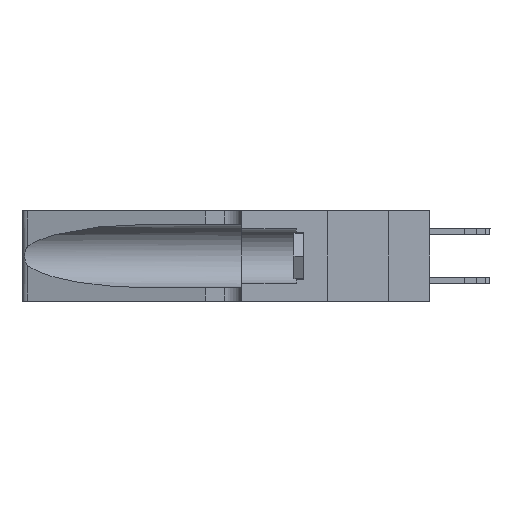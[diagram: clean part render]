
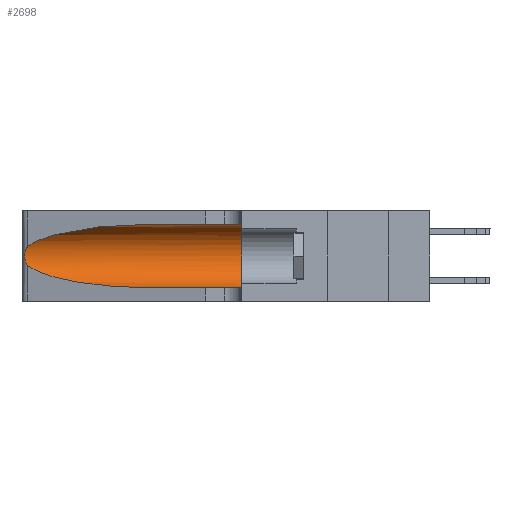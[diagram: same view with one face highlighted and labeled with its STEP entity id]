
A CAD part, left-side view. The second image highlights one B-rep face of the part: STEP entity #2698.
In plain terms, the highlighted cylindrical face has radius 3.308 mm (diameter 6.617 mm), a partial arc.
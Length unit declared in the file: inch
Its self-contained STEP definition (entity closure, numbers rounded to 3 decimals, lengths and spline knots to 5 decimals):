
#829 = CARTESIAN_POINT ( 'NONE',  ( 0.25487, 1.22718, 0.14631 ) ) ;
#1090 = CARTESIAN_POINT ( 'NONE',  ( 0.26075, 1.23896, 0.19203 ) ) ;
#1494 = CARTESIAN_POINT ( 'NONE',  ( 0.18966, 0.96281, 0.31525 ) ) ;
#1847 = VERTEX_POINT ( 'NONE', #18610 ) ;
#1973 = DIRECTION ( 'NONE',  ( 0., 1., 0. ) ) ;
#2018 = ORIENTED_EDGE ( 'NONE', *, *, #15554, .T. ) ;
#2055 = EDGE_CURVE ( 'NONE', #8848, #1847, #17939, .T. ) ;
#2092 = EDGE_CURVE ( 'NONE', #1847, #3056, #12847, .T. ) ;
#2271 =( BOUNDED_CURVE ( )  B_SPLINE_CURVE ( 3, ( #7431, #12796, #12648, #5830 ),
 .UNSPECIFIED., .F., .F. ) 
 B_SPLINE_CURVE_WITH_KNOTS ( ( 4, 4 ),
 ( 3.44316, 4.71239 ),
 .UNSPECIFIED. ) 
 CURVE ( )  GEOMETRIC_REPRESENTATION_ITEM ( )  RATIONAL_B_SPLINE_CURVE ( ( 1., 0.87, 0.87, 1. ) ) 
 REPRESENTATION_ITEM ( '' )  );
#2698 = ADVANCED_FACE ( 'NONE', ( #14183 ), #19706, .F. ) ;
#2825 = ORIENTED_EDGE ( 'NONE', *, *, #3946, .T. ) ;
#3056 = VERTEX_POINT ( 'NONE', #829 ) ;
#3180 = DIRECTION ( 'NONE',  ( 0., -1., 0. ) ) ;
#3276 = CARTESIAN_POINT ( 'NONE',  ( 0.1305, 1.61858, 0.05475 ) ) ;
#3824 = CARTESIAN_POINT ( 'NONE',  ( 0.1305, 0.35, 0.185 ) ) ;
#3946 = EDGE_CURVE ( 'NONE', #22287, #8185, #4849, .T. ) ;
#3987 = VECTOR ( 'NONE', #6839, 39.37008 ) ;
#4849 = LINE ( 'NONE', #3276, #3987 ) ;
#4854 = CARTESIAN_POINT ( 'NONE',  ( 0.25639, 1.23184, 0.21858 ) ) ;
#5127 = AXIS2_PLACEMENT_3D ( 'NONE', #3824, #1973, #7308 ) ;
#5688 = EDGE_LOOP ( 'NONE', ( #17604, #20027, #2018, #2825, #14156, #18607 ) ) ;
#5733 = CARTESIAN_POINT ( 'NONE',  ( 0.25487, 1.22718, 0.22369 ) ) ;
#5830 = CARTESIAN_POINT ( 'NONE',  ( 0.1305, 0.72297, 0.05475 ) ) ;
#6083 = CARTESIAN_POINT ( 'NONE',  ( 0.1305, 0.35, 0.05475 ) ) ;
#6839 = DIRECTION ( 'NONE',  ( 0., -1., 0. ) ) ;
#7308 = DIRECTION ( 'NONE',  ( 0., 0., 1. ) ) ;
#7431 = CARTESIAN_POINT ( 'NONE',  ( 0.25487, 1.22718, 0.14631 ) ) ;
#7936 = LINE ( 'NONE', #16104, #18364 ) ;
#8185 = VERTEX_POINT ( 'NONE', #6083 ) ;
#8848 = VERTEX_POINT ( 'NONE', #9189 ) ;
#9189 = CARTESIAN_POINT ( 'NONE',  ( 0.1305, 0.72297, 0.31525 ) ) ;
#9235 = DIRECTION ( 'NONE',  ( 0., -1., 0. ) ) ;
#9632 = CARTESIAN_POINT ( 'NONE',  ( 0.25555, 1.22994, 0.2215 ) ) ;
#9934 = VERTEX_POINT ( 'NONE', #15305 ) ;
#10336 = CARTESIAN_POINT ( 'NONE',  ( 0.1305, 1.61858, 0.185 ) ) ;
#10504 = CARTESIAN_POINT ( 'NONE',  ( 0.25487, 1.22718, 0.22369 ) ) ;
#12648 = CARTESIAN_POINT ( 'NONE',  ( 0.18966, 0.96281, 0.05475 ) ) ;
#12796 = CARTESIAN_POINT ( 'NONE',  ( 0.2373, 1.15595, 0.08982 ) ) ;
#12847 = B_SPLINE_CURVE_WITH_KNOTS ( 'NONE', 3,
 ( #5733, #9632, #4854, #17564, #18334, #22196, #1090, #15235, #17013, #17481, #20920, #21816, #19718, #22550 ),
 .UNSPECIFIED., .F., .F.,
 ( 4, 2, 2, 2, 2, 2, 4 ),
 ( 0., 0.00027, 0.00053, 0.00107, 0.0016, 0.00187, 0.00214 ),
 .UNSPECIFIED. ) ;
#13358 = CIRCLE ( 'NONE', #5127, 0.13025 ) ;
#14156 = ORIENTED_EDGE ( 'NONE', *, *, #19240, .F. ) ;
#14183 = FACE_OUTER_BOUND ( 'NONE', #5688, .T. ) ;
#15235 = CARTESIAN_POINT ( 'NONE',  ( 0.26075, 1.23896, 0.178 ) ) ;
#15305 = CARTESIAN_POINT ( 'NONE',  ( 0.1305, 0.35, 0.31525 ) ) ;
#15554 = EDGE_CURVE ( 'NONE', #3056, #22287, #2271, .T. ) ;
#16104 = CARTESIAN_POINT ( 'NONE',  ( 0.1305, 1.61858, 0.31525 ) ) ;
#16675 = CARTESIAN_POINT ( 'NONE',  ( 0.1305, 0.72297, 0.05475 ) ) ;
#17013 = CARTESIAN_POINT ( 'NONE',  ( 0.26017, 1.23833, 0.17102 ) ) ;
#17336 = CARTESIAN_POINT ( 'NONE',  ( 0.2373, 1.15595, 0.28018 ) ) ;
#17481 = CARTESIAN_POINT ( 'NONE',  ( 0.25856, 1.23593, 0.16098 ) ) ;
#17564 = CARTESIAN_POINT ( 'NONE',  ( 0.25787, 1.23484, 0.2124 ) ) ;
#17604 = ORIENTED_EDGE ( 'NONE', *, *, #2055, .T. ) ;
#17646 = AXIS2_PLACEMENT_3D ( 'NONE', #10336, #3180, #20552 ) ;
#17939 =( BOUNDED_CURVE ( )  B_SPLINE_CURVE ( 3, ( #21039, #1494, #17336, #10504 ),
 .UNSPECIFIED., .F., .F. ) 
 B_SPLINE_CURVE_WITH_KNOTS ( ( 4, 4 ),
 ( 1.5708, 2.84003 ),
 .UNSPECIFIED. ) 
 CURVE ( )  GEOMETRIC_REPRESENTATION_ITEM ( )  RATIONAL_B_SPLINE_CURVE ( ( 1., 0.87, 0.87, 1. ) ) 
 REPRESENTATION_ITEM ( '' )  );
#18334 = CARTESIAN_POINT ( 'NONE',  ( 0.25854, 1.2359, 0.20912 ) ) ;
#18364 = VECTOR ( 'NONE', #9235, 39.37008 ) ;
#18607 = ORIENTED_EDGE ( 'NONE', *, *, #20918, .F. ) ;
#18610 = CARTESIAN_POINT ( 'NONE',  ( 0.25487, 1.22718, 0.22369 ) ) ;
#19240 = EDGE_CURVE ( 'NONE', #9934, #8185, #13358, .T. ) ;
#19706 = CYLINDRICAL_SURFACE ( 'NONE', #17646, 0.13025 ) ;
#19718 = CARTESIAN_POINT ( 'NONE',  ( 0.25555, 1.22993, 0.14849 ) ) ;
#20027 = ORIENTED_EDGE ( 'NONE', *, *, #2092, .T. ) ;
#20552 = DIRECTION ( 'NONE',  ( 0., 0., -1. ) ) ;
#20918 = EDGE_CURVE ( 'NONE', #8848, #9934, #7936, .T. ) ;
#20920 = CARTESIAN_POINT ( 'NONE',  ( 0.25789, 1.23486, 0.15765 ) ) ;
#21039 = CARTESIAN_POINT ( 'NONE',  ( 0.1305, 0.72297, 0.31525 ) ) ;
#21816 = CARTESIAN_POINT ( 'NONE',  ( 0.25639, 1.23186, 0.15144 ) ) ;
#22196 = CARTESIAN_POINT ( 'NONE',  ( 0.26018, 1.23835, 0.19895 ) ) ;
#22287 = VERTEX_POINT ( 'NONE', #16675 ) ;
#22550 = CARTESIAN_POINT ( 'NONE',  ( 0.25487, 1.22718, 0.14631 ) ) ;
